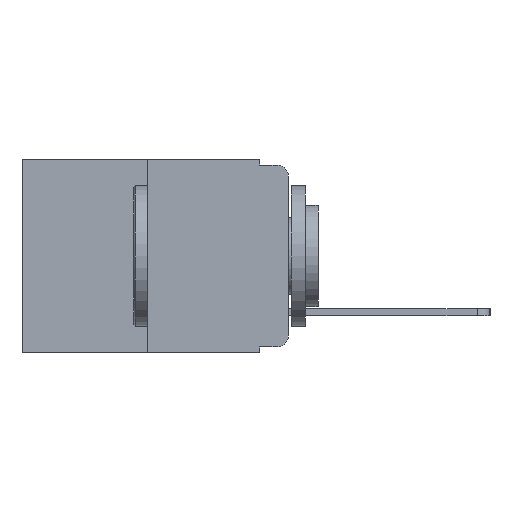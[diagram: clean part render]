
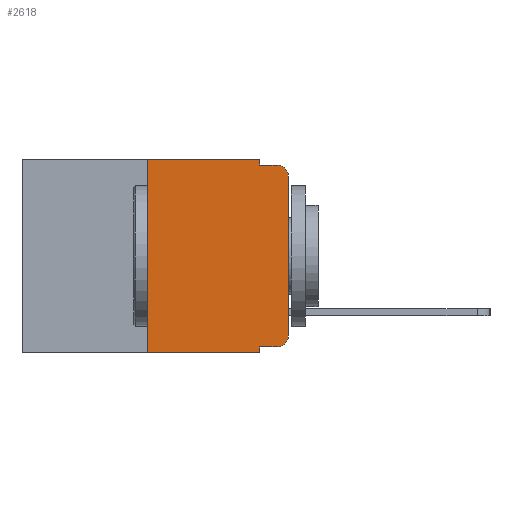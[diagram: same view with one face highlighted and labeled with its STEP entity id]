
A CAD part, left-side view. The second image highlights one B-rep face of the part: STEP entity #2618.
In plain terms, the highlighted planar face has unit normal (-1, 0, 0).
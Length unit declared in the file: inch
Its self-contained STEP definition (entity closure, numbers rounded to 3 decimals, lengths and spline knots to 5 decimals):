
#28 = VECTOR ( 'NONE', #3335, 39.37008 ) ;
#53 = VERTEX_POINT ( 'NONE', #2079 ) ;
#263 = CIRCLE ( 'NONE', #12371, 0.02 ) ;
#800 = VECTOR ( 'NONE', #1782, 39.37008 ) ;
#809 = EDGE_CURVE ( 'NONE', #9290, #3254, #11020, .T. ) ;
#920 = CARTESIAN_POINT ( 'NONE',  ( 0., 0.051, -0.01 ) ) ;
#972 = LINE ( 'NONE', #13329, #9474 ) ;
#999 = EDGE_CURVE ( 'NONE', #9488, #10175, #9249, .T. ) ;
#1115 = LINE ( 'NONE', #13445, #12970 ) ;
#1185 = ORIENTED_EDGE ( 'NONE', *, *, #11006, .F. ) ;
#1186 = EDGE_CURVE ( 'NONE', #2473, #9875, #1115, .T. ) ;
#1198 = EDGE_CURVE ( 'NONE', #6973, #1945, #7306, .T. ) ;
#1465 = ORIENTED_EDGE ( 'NONE', *, *, #11301, .T. ) ;
#1590 = DIRECTION ( 'NONE',  ( 0., -1., 0. ) ) ;
#1676 = CARTESIAN_POINT ( 'NONE',  ( 0., 0., -0.03 ) ) ;
#1734 = DIRECTION ( 'NONE',  ( -1., 0., 0. ) ) ;
#1782 = DIRECTION ( 'NONE',  ( 0., 0., 1. ) ) ;
#1801 = LINE ( 'NONE', #5244, #5235 ) ;
#1945 = VERTEX_POINT ( 'NONE', #3851 ) ;
#2079 = CARTESIAN_POINT ( 'NONE',  ( 0., 0., -0.313 ) ) ;
#2276 = CARTESIAN_POINT ( 'NONE',  ( 0., 0.051, -0.333 ) ) ;
#2444 = EDGE_CURVE ( 'NONE', #9875, #9488, #1801, .T. ) ;
#2473 = VERTEX_POINT ( 'NONE', #4937 ) ;
#2618 = ADVANCED_FACE ( 'NONE', ( #14492 ), #6532, .F. ) ;
#2660 = ORIENTED_EDGE ( 'NONE', *, *, #2444, .F. ) ;
#2754 = CARTESIAN_POINT ( 'NONE',  ( 0., 0.473, 0. ) ) ;
#2839 = EDGE_LOOP ( 'NONE', ( #5739, #4989, #3249, #2660, #10252, #1185, #6886, #6836, #14084, #1465 ) ) ;
#3249 = ORIENTED_EDGE ( 'NONE', *, *, #999, .F. ) ;
#3254 = VERTEX_POINT ( 'NONE', #13633 ) ;
#3335 = DIRECTION ( 'NONE',  ( 0., -1., 0. ) ) ;
#3606 = CARTESIAN_POINT ( 'NONE',  ( 0., 0.02, -0.01 ) ) ;
#3851 = CARTESIAN_POINT ( 'NONE',  ( 0., 0.02, -0.333 ) ) ;
#4498 = DIRECTION ( 'NONE',  ( 0., 0., 1. ) ) ;
#4937 = CARTESIAN_POINT ( 'NONE',  ( 0., 0.25, 0. ) ) ;
#4989 = ORIENTED_EDGE ( 'NONE', *, *, #5562, .T. ) ;
#5045 = AXIS2_PLACEMENT_3D ( 'NONE', #2754, #7351, #6934 ) ;
#5235 = VECTOR ( 'NONE', #5266, 39.37008 ) ;
#5244 = CARTESIAN_POINT ( 'NONE',  ( 0., 0.051, 0. ) ) ;
#5266 = DIRECTION ( 'NONE',  ( 0., 0., -1. ) ) ;
#5562 = EDGE_CURVE ( 'NONE', #12528, #10175, #11974, .T. ) ;
#5643 = EDGE_CURVE ( 'NONE', #53, #12528, #972, .T. ) ;
#5739 = ORIENTED_EDGE ( 'NONE', *, *, #5643, .T. ) ;
#6350 = CARTESIAN_POINT ( 'NONE',  ( 0., 0.02, -0.03 ) ) ;
#6532 = PLANE ( 'NONE',  #5045 ) ;
#6597 = LINE ( 'NONE', #9876, #800 ) ;
#6836 = ORIENTED_EDGE ( 'NONE', *, *, #13225, .F. ) ;
#6886 = ORIENTED_EDGE ( 'NONE', *, *, #809, .T. ) ;
#6897 = DIRECTION ( 'NONE',  ( -1., 0., 0. ) ) ;
#6932 = VECTOR ( 'NONE', #1590, 39.37008 ) ;
#6934 = DIRECTION ( 'NONE',  ( 0., 0., -1. ) ) ;
#6973 = VERTEX_POINT ( 'NONE', #14233 ) ;
#7306 = LINE ( 'NONE', #2276, #6932 ) ;
#7351 = DIRECTION ( 'NONE',  ( 1., 0., 0. ) ) ;
#7414 = DIRECTION ( 'NONE',  ( 0., -1., 0. ) ) ;
#7488 = LINE ( 'NONE', #11322, #13138 ) ;
#8015 = VECTOR ( 'NONE', #8414, 39.37008 ) ;
#8414 = DIRECTION ( 'NONE',  ( 0., -1., 0. ) ) ;
#8937 = CARTESIAN_POINT ( 'NONE',  ( 0., 0.473, -0.343 ) ) ;
#9249 = LINE ( 'NONE', #920, #28 ) ;
#9290 = VERTEX_POINT ( 'NONE', #13160 ) ;
#9468 = DIRECTION ( 'NONE',  ( 0., 0., -1. ) ) ;
#9474 = VECTOR ( 'NONE', #4498, 39.37008 ) ;
#9488 = VERTEX_POINT ( 'NONE', #13586 ) ;
#9875 = VERTEX_POINT ( 'NONE', #14555 ) ;
#9876 = CARTESIAN_POINT ( 'NONE',  ( 0., 0.25, 0. ) ) ;
#10175 = VERTEX_POINT ( 'NONE', #3606 ) ;
#10217 = AXIS2_PLACEMENT_3D ( 'NONE', #6350, #1734, #9468 ) ;
#10252 = ORIENTED_EDGE ( 'NONE', *, *, #1186, .F. ) ;
#11006 = EDGE_CURVE ( 'NONE', #9290, #2473, #6597, .T. ) ;
#11020 = LINE ( 'NONE', #8937, #8015 ) ;
#11301 = EDGE_CURVE ( 'NONE', #1945, #53, #263, .T. ) ;
#11322 = CARTESIAN_POINT ( 'NONE',  ( 0., 0.051, 0. ) ) ;
#11974 = CIRCLE ( 'NONE', #10217, 0.02 ) ;
#12371 = AXIS2_PLACEMENT_3D ( 'NONE', #13679, #6897, #14792 ) ;
#12459 = DIRECTION ( 'NONE',  ( 0., 0., -1. ) ) ;
#12528 = VERTEX_POINT ( 'NONE', #1676 ) ;
#12970 = VECTOR ( 'NONE', #7414, 39.37008 ) ;
#13138 = VECTOR ( 'NONE', #12459, 39.37008 ) ;
#13160 = CARTESIAN_POINT ( 'NONE',  ( 0., 0.25, -0.343 ) ) ;
#13225 = EDGE_CURVE ( 'NONE', #6973, #3254, #7488, .T. ) ;
#13329 = CARTESIAN_POINT ( 'NONE',  ( 0., 0., 0. ) ) ;
#13445 = CARTESIAN_POINT ( 'NONE',  ( 0., 0.473, 0. ) ) ;
#13586 = CARTESIAN_POINT ( 'NONE',  ( 0., 0.051, -0.01 ) ) ;
#13633 = CARTESIAN_POINT ( 'NONE',  ( 0., 0.051, -0.343 ) ) ;
#13679 = CARTESIAN_POINT ( 'NONE',  ( 0., 0.02, -0.313 ) ) ;
#14084 = ORIENTED_EDGE ( 'NONE', *, *, #1198, .T. ) ;
#14233 = CARTESIAN_POINT ( 'NONE',  ( 0., 0.051, -0.333 ) ) ;
#14492 = FACE_OUTER_BOUND ( 'NONE', #2839, .T. ) ;
#14555 = CARTESIAN_POINT ( 'NONE',  ( 0., 0.051, 0. ) ) ;
#14792 = DIRECTION ( 'NONE',  ( 0., 0., -1. ) ) ;
